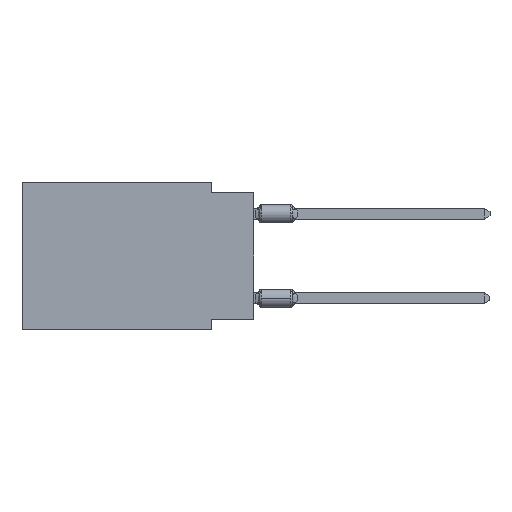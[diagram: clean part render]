
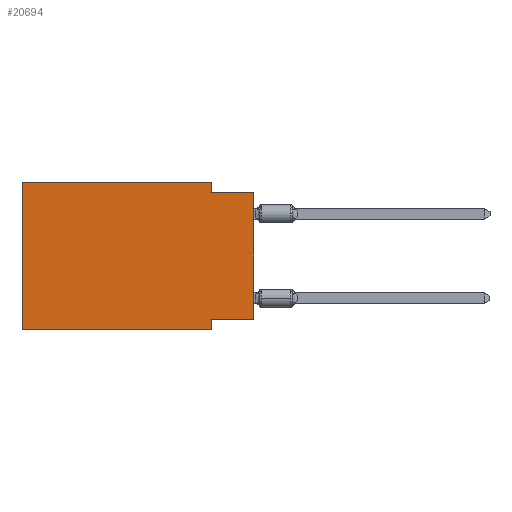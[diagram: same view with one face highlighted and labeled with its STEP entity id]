
A CAD part, left-side view. The second image highlights one B-rep face of the part: STEP entity #20694.
In plain terms, the highlighted planar face has unit normal (-1, 0, 0).
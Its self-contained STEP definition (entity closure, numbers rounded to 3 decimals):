
#59 = EDGE_CURVE ( 'NONE', #23048, #21043, #7567, .T. ) ;
#189 = EDGE_CURVE ( 'NONE', #28127, #5216, #7182, .T. ) ;
#417 = DIRECTION ( 'NONE',  ( 0., 0., -1. ) ) ;
#491 = CARTESIAN_POINT ( 'NONE',  ( 0., 2.54, -0.635 ) ) ;
#710 = VERTEX_POINT ( 'NONE', #17335 ) ;
#854 = VECTOR ( 'NONE', #3236, 1000. ) ;
#1001 = ORIENTED_EDGE ( 'NONE', *, *, #7142, .F. ) ;
#1462 = DIRECTION ( 'NONE',  ( 0., -1., 0. ) ) ;
#2774 = FACE_OUTER_BOUND ( 'NONE', #9017, .T. ) ;
#2955 = ORIENTED_EDGE ( 'NONE', *, *, #20381, .F. ) ;
#3189 = DIRECTION ( 'NONE',  ( 0., 0., 1. ) ) ;
#3236 = DIRECTION ( 'NONE',  ( 0., -1., 0. ) ) ;
#3959 = ORIENTED_EDGE ( 'NONE', *, *, #189, .F. ) ;
#4990 = DIRECTION ( 'NONE',  ( 0., 0., -1. ) ) ;
#5216 = VERTEX_POINT ( 'NONE', #20142 ) ;
#5916 = VECTOR ( 'NONE', #4990, 1000. ) ;
#6006 = LINE ( 'NONE', #23980, #22352 ) ;
#6360 = EDGE_CURVE ( 'NONE', #8863, #12646, #28346, .T. ) ;
#7142 = EDGE_CURVE ( 'NONE', #18334, #12646, #19214, .T. ) ;
#7182 = LINE ( 'NONE', #16099, #5916 ) ;
#7473 = LINE ( 'NONE', #22964, #854 ) ;
#7567 = LINE ( 'NONE', #16486, #8717 ) ;
#7591 = VECTOR ( 'NONE', #10299, 1000. ) ;
#8717 = VECTOR ( 'NONE', #3189, 1000. ) ;
#8863 = VERTEX_POINT ( 'NONE', #23965 ) ;
#9017 = EDGE_LOOP ( 'NONE', ( #27972, #1001, #21153, #2955, #25073, #16289, #3959, #27365 ) ) ;
#9377 = VECTOR ( 'NONE', #14339, 1000. ) ;
#10299 = DIRECTION ( 'NONE',  ( 0., -1., 0. ) ) ;
#10777 = LINE ( 'NONE', #15457, #26846 ) ;
#10827 = CARTESIAN_POINT ( 'NONE',  ( 0., 2.54, -8.255 ) ) ;
#11069 = DIRECTION ( 'NONE',  ( 0., 0., -1. ) ) ;
#11705 = CARTESIAN_POINT ( 'NONE',  ( 0., 13.97, 0. ) ) ;
#12529 = EDGE_CURVE ( 'NONE', #8863, #28127, #19347, .T. ) ;
#12646 = VERTEX_POINT ( 'NONE', #23578 ) ;
#14038 = PLANE ( 'NONE',  #27032 ) ;
#14339 = DIRECTION ( 'NONE',  ( 0., 0., 1. ) ) ;
#14972 = CARTESIAN_POINT ( 'NONE',  ( 0., 0., -8.255 ) ) ;
#15457 = CARTESIAN_POINT ( 'NONE',  ( 0., 2.54, 0. ) ) ;
#15847 = CARTESIAN_POINT ( 'NONE',  ( 0., 13.97, -8.89 ) ) ;
#16099 = CARTESIAN_POINT ( 'NONE',  ( 0., 2.54, -8.89 ) ) ;
#16215 = DIRECTION ( 'NONE',  ( 1., 0., 0. ) ) ;
#16289 = ORIENTED_EDGE ( 'NONE', *, *, #20355, .T. ) ;
#16486 = CARTESIAN_POINT ( 'NONE',  ( 0., 13.97, 0. ) ) ;
#17335 = CARTESIAN_POINT ( 'NONE',  ( 0., 2.54, 0. ) ) ;
#17515 = CARTESIAN_POINT ( 'NONE',  ( 0., 13.97, 0. ) ) ;
#18334 = VERTEX_POINT ( 'NONE', #491 ) ;
#19214 = LINE ( 'NONE', #25775, #7591 ) ;
#19347 = LINE ( 'NONE', #14972, #25588 ) ;
#20142 = CARTESIAN_POINT ( 'NONE',  ( 0., 2.54, -8.89 ) ) ;
#20355 = EDGE_CURVE ( 'NONE', #23048, #5216, #7473, .T. ) ;
#20381 = EDGE_CURVE ( 'NONE', #21043, #710, #6006, .T. ) ;
#20694 = ADVANCED_FACE ( 'NONE', ( #2774 ), #14038, .F. ) ;
#21043 = VERTEX_POINT ( 'NONE', #17515 ) ;
#21153 = ORIENTED_EDGE ( 'NONE', *, *, #21322, .F. ) ;
#21322 = EDGE_CURVE ( 'NONE', #710, #18334, #10777, .T. ) ;
#22352 = VECTOR ( 'NONE', #1462, 1000. ) ;
#22964 = CARTESIAN_POINT ( 'NONE',  ( 0., 13.97, -8.89 ) ) ;
#23048 = VERTEX_POINT ( 'NONE', #15847 ) ;
#23578 = CARTESIAN_POINT ( 'NONE',  ( 0., 0., -0.635 ) ) ;
#23965 = CARTESIAN_POINT ( 'NONE',  ( 0., 0., -8.255 ) ) ;
#23980 = CARTESIAN_POINT ( 'NONE',  ( 0., 13.97, 0. ) ) ;
#25073 = ORIENTED_EDGE ( 'NONE', *, *, #59, .F. ) ;
#25588 = VECTOR ( 'NONE', #28106, 1000. ) ;
#25775 = CARTESIAN_POINT ( 'NONE',  ( 0., 0., -0.635 ) ) ;
#26167 = CARTESIAN_POINT ( 'NONE',  ( 0., 0., 0. ) ) ;
#26846 = VECTOR ( 'NONE', #11069, 1000. ) ;
#27032 = AXIS2_PLACEMENT_3D ( 'NONE', #11705, #16215, #417 ) ;
#27365 = ORIENTED_EDGE ( 'NONE', *, *, #12529, .F. ) ;
#27972 = ORIENTED_EDGE ( 'NONE', *, *, #6360, .T. ) ;
#28106 = DIRECTION ( 'NONE',  ( 0., 1., 0. ) ) ;
#28127 = VERTEX_POINT ( 'NONE', #10827 ) ;
#28346 = LINE ( 'NONE', #26167, #9377 ) ;
